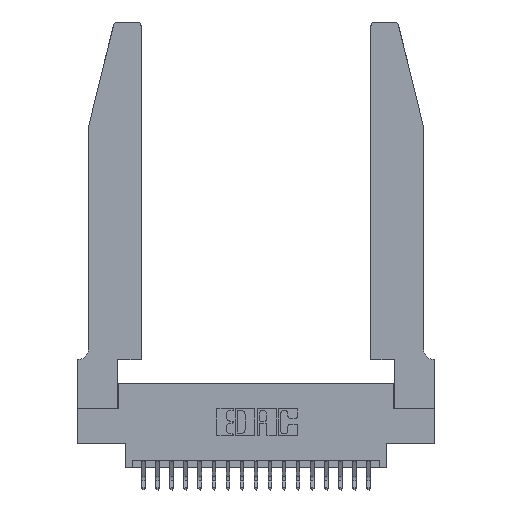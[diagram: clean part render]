
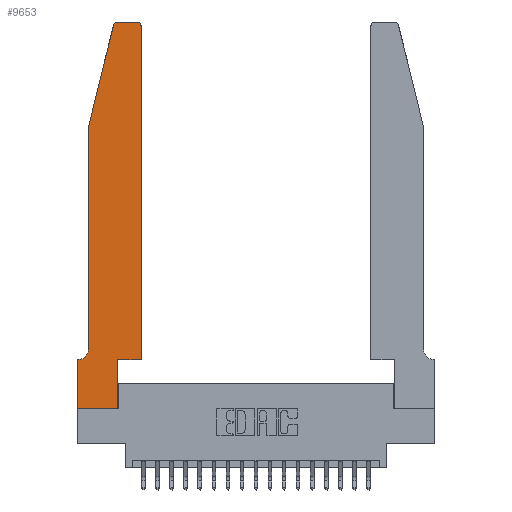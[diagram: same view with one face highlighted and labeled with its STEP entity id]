
A CAD part, top view. The second image highlights one B-rep face of the part: STEP entity #9653.
In plain terms, the highlighted planar face has unit normal (0, 0, 1).
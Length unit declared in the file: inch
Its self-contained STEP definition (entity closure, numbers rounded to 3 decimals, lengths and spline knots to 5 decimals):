
#93 = CARTESIAN_POINT ( 'NONE',  ( 0.4205, 2.75, 0.37 ) ) ;
#367 = VERTEX_POINT ( 'NONE', #8940 ) ;
#580 = EDGE_CURVE ( 'NONE', #9620, #5906, #7136, .T. ) ;
#602 = LINE ( 'NONE', #21387, #17973 ) ;
#666 = EDGE_CURVE ( 'NONE', #1382, #15757, #12424, .T. ) ;
#865 = EDGE_CURVE ( 'NONE', #8061, #367, #13741, .T. ) ;
#919 = CARTESIAN_POINT ( 'NONE',  ( 0.284, 2.72, 0.37 ) ) ;
#1023 = LINE ( 'NONE', #18512, #13952 ) ;
#1138 = DIRECTION ( 'NONE',  ( 0., 0., -1. ) ) ;
#1371 = DIRECTION ( 'NONE',  ( 0., 0., 1. ) ) ;
#1382 = VERTEX_POINT ( 'NONE', #15112 ) ;
#1658 = VERTEX_POINT ( 'NONE', #7355 ) ;
#1815 = VECTOR ( 'NONE', #1866, 39.37008 ) ;
#1866 = DIRECTION ( 'NONE',  ( 0., 1., 0. ) ) ;
#2028 = ORIENTED_EDGE ( 'NONE', *, *, #9420, .T. ) ;
#2242 = ORIENTED_EDGE ( 'NONE', *, *, #13389, .T. ) ;
#2395 = DIRECTION ( 'NONE',  ( 0., 0., 1. ) ) ;
#2400 = VECTOR ( 'NONE', #8214, 39.37008 ) ;
#2489 = ORIENTED_EDGE ( 'NONE', *, *, #2632, .T. ) ;
#2584 = VECTOR ( 'NONE', #14042, 39.37008 ) ;
#2632 = EDGE_CURVE ( 'NONE', #11005, #1382, #8361, .T. ) ;
#2793 = LINE ( 'NONE', #14334, #15195 ) ;
#2907 = CARTESIAN_POINT ( 'NONE',  ( 0.284, 2.75, 0.37 ) ) ;
#3346 = ORIENTED_EDGE ( 'NONE', *, *, #865, .T. ) ;
#3579 = EDGE_CURVE ( 'NONE', #21492, #15181, #19731, .T. ) ;
#3926 = VERTEX_POINT ( 'NONE', #9669 ) ;
#4647 = CARTESIAN_POINT ( 'NONE',  ( 0.25487, 2.72718, 0.37 ) ) ;
#4666 = LINE ( 'NONE', #17238, #2584 ) ;
#5871 = DIRECTION ( 'NONE',  ( 0., 0., 1. ) ) ;
#5906 = VERTEX_POINT ( 'NONE', #4647 ) ;
#6217 = CARTESIAN_POINT ( 'NONE',  ( 0., 0.35, 0.37 ) ) ;
#6357 = DIRECTION ( 'NONE',  ( 1., 0., 0. ) ) ;
#6903 = CARTESIAN_POINT ( 'NONE',  ( 0.2865, 0.35, 0.37 ) ) ;
#6915 = CARTESIAN_POINT ( 'NONE',  ( 0.2865, 0.35, 0.37 ) ) ;
#6918 = VECTOR ( 'NONE', #21058, 39.37008 ) ;
#7059 = FACE_OUTER_BOUND ( 'NONE', #17123, .T. ) ;
#7136 = CIRCLE ( 'NONE', #8069, 0.03 ) ;
#7163 = CARTESIAN_POINT ( 'NONE',  ( 0.0755, 2., 0.37 ) ) ;
#7355 = CARTESIAN_POINT ( 'NONE',  ( 0.4505, 2.72, 0.37 ) ) ;
#7711 = ORIENTED_EDGE ( 'NONE', *, *, #13951, .T. ) ;
#7911 = VECTOR ( 'NONE', #21229, 39.37008 ) ;
#8061 = VERTEX_POINT ( 'NONE', #16758 ) ;
#8069 = AXIS2_PLACEMENT_3D ( 'NONE', #919, #2395, #12708 ) ;
#8214 = DIRECTION ( 'NONE',  ( 1., 0., 0. ) ) ;
#8361 = CIRCLE ( 'NONE', #11219, 0.07 ) ;
#8940 = CARTESIAN_POINT ( 'NONE',  ( 0.2865, 0., 0.37 ) ) ;
#9295 = CARTESIAN_POINT ( 'NONE',  ( 0.0055, 0.42, 0.37 ) ) ;
#9420 = EDGE_CURVE ( 'NONE', #15181, #1658, #4666, .T. ) ;
#9620 = VERTEX_POINT ( 'NONE', #2907 ) ;
#9653 = ADVANCED_FACE ( 'NONE', ( #7059 ), #19793, .T. ) ;
#9669 = CARTESIAN_POINT ( 'NONE',  ( 0.0755, 2., 0.37 ) ) ;
#9791 = DIRECTION ( 'NONE',  ( 0., -1., 0. ) ) ;
#9916 = CARTESIAN_POINT ( 'NONE',  ( 0.0755, 0.42, 0.37 ) ) ;
#10492 = CARTESIAN_POINT ( 'NONE',  ( 0., 0.35, 0.37 ) ) ;
#11005 = VERTEX_POINT ( 'NONE', #9916 ) ;
#11204 = EDGE_CURVE ( 'NONE', #3926, #11005, #2793, .T. ) ;
#11219 = AXIS2_PLACEMENT_3D ( 'NONE', #9295, #1138, #11301 ) ;
#11301 = DIRECTION ( 'NONE',  ( -1., 0., 0. ) ) ;
#11423 = AXIS2_PLACEMENT_3D ( 'NONE', #15972, #5871, #19373 ) ;
#11980 = CIRCLE ( 'NONE', #11423, 0.03 ) ;
#12178 = AXIS2_PLACEMENT_3D ( 'NONE', #6217, #1371, #6357 ) ;
#12424 = LINE ( 'NONE', #12821, #7911 ) ;
#12708 = DIRECTION ( 'NONE',  ( 1., 0., 0. ) ) ;
#12821 = CARTESIAN_POINT ( 'NONE',  ( 0.0755, 0.35, 0.37 ) ) ;
#13325 = ORIENTED_EDGE ( 'NONE', *, *, #580, .T. ) ;
#13389 = EDGE_CURVE ( 'NONE', #1658, #21776, #11980, .T. ) ;
#13741 = LINE ( 'NONE', #20184, #2400 ) ;
#13951 = EDGE_CURVE ( 'NONE', #5906, #3926, #16427, .T. ) ;
#13952 = VECTOR ( 'NONE', #20214, 39.37008 ) ;
#14042 = DIRECTION ( 'NONE',  ( 0., 1., 0. ) ) ;
#14334 = CARTESIAN_POINT ( 'NONE',  ( 0.0755, 2., 0.37 ) ) ;
#15112 = CARTESIAN_POINT ( 'NONE',  ( 0.0055, 0.35, 0.37 ) ) ;
#15181 = VERTEX_POINT ( 'NONE', #17679 ) ;
#15195 = VECTOR ( 'NONE', #17734, 39.37008 ) ;
#15676 = ORIENTED_EDGE ( 'NONE', *, *, #16627, .T. ) ;
#15757 = VERTEX_POINT ( 'NONE', #10492 ) ;
#15860 = ORIENTED_EDGE ( 'NONE', *, *, #16560, .T. ) ;
#15972 = CARTESIAN_POINT ( 'NONE',  ( 0.4205, 2.72, 0.37 ) ) ;
#16298 = ORIENTED_EDGE ( 'NONE', *, *, #3579, .T. ) ;
#16427 = LINE ( 'NONE', #7163, #6918 ) ;
#16560 = EDGE_CURVE ( 'NONE', #21776, #9620, #1023, .T. ) ;
#16627 = EDGE_CURVE ( 'NONE', #367, #21492, #18683, .T. ) ;
#16758 = CARTESIAN_POINT ( 'NONE',  ( 0., 0., 0.37 ) ) ;
#17123 = EDGE_LOOP ( 'NONE', ( #15860, #13325, #7711, #17487, #2489, #19839, #19417, #3346, #15676, #16298, #2028, #2242 ) ) ;
#17238 = CARTESIAN_POINT ( 'NONE',  ( 0.4505, 0.35, 0.37 ) ) ;
#17429 = DIRECTION ( 'NONE',  ( 1., 0., 0. ) ) ;
#17487 = ORIENTED_EDGE ( 'NONE', *, *, #11204, .T. ) ;
#17679 = CARTESIAN_POINT ( 'NONE',  ( 0.4505, 0.35, 0.37 ) ) ;
#17734 = DIRECTION ( 'NONE',  ( 0., -1., 0. ) ) ;
#17973 = VECTOR ( 'NONE', #9791, 39.37008 ) ;
#18512 = CARTESIAN_POINT ( 'NONE',  ( 0.2605, 2.75, 0.37 ) ) ;
#18675 = VECTOR ( 'NONE', #17429, 39.37008 ) ;
#18683 = LINE ( 'NONE', #6915, #1815 ) ;
#19183 = CARTESIAN_POINT ( 'NONE',  ( 0.4505, 0.35, 0.37 ) ) ;
#19373 = DIRECTION ( 'NONE',  ( 1., 0., 0. ) ) ;
#19417 = ORIENTED_EDGE ( 'NONE', *, *, #20209, .T. ) ;
#19731 = LINE ( 'NONE', #19183, #18675 ) ;
#19793 = PLANE ( 'NONE',  #12178 ) ;
#19839 = ORIENTED_EDGE ( 'NONE', *, *, #666, .T. ) ;
#20184 = CARTESIAN_POINT ( 'NONE',  ( 0., 0., 0.37 ) ) ;
#20209 = EDGE_CURVE ( 'NONE', #15757, #8061, #602, .T. ) ;
#20214 = DIRECTION ( 'NONE',  ( -1., 0., 0. ) ) ;
#21058 = DIRECTION ( 'NONE',  ( -0.239, -0.971, 0. ) ) ;
#21229 = DIRECTION ( 'NONE',  ( -1., 0., 0. ) ) ;
#21387 = CARTESIAN_POINT ( 'NONE',  ( 0., 0., 0.37 ) ) ;
#21492 = VERTEX_POINT ( 'NONE', #6903 ) ;
#21776 = VERTEX_POINT ( 'NONE', #93 ) ;
